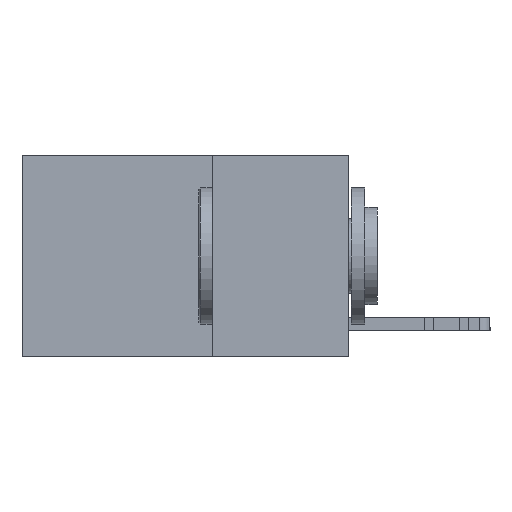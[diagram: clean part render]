
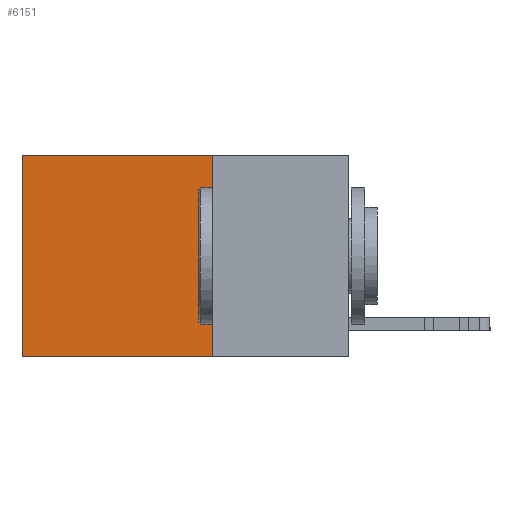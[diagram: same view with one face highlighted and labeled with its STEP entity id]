
A CAD part, left-side view. The second image highlights one B-rep face of the part: STEP entity #6151.
In plain terms, the highlighted planar face has unit normal (-1, 0, 0).
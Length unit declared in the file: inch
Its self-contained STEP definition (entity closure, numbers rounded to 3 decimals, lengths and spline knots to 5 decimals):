
#1271 = VERTEX_POINT ( 'NONE', #16680 ) ;
#1793 = EDGE_CURVE ( 'NONE', #1271, #24748, #17852, .T. ) ;
#2706 = FACE_OUTER_BOUND ( 'NONE', #16881, .T. ) ;
#2847 = VECTOR ( 'NONE', #13712, 39.37008 ) ;
#3685 = CARTESIAN_POINT ( 'NONE',  ( 0.2625, 0.25, -0.37 ) ) ;
#4338 = VECTOR ( 'NONE', #7626, 39.37008 ) ;
#4457 = CARTESIAN_POINT ( 'NONE',  ( 0.2625, 0.25, -0.37 ) ) ;
#5305 = CARTESIAN_POINT ( 'NONE',  ( 0.2625, 0.25, 0. ) ) ;
#6151 = ADVANCED_FACE ( 'NONE', ( #2706 ), #21548, .F. ) ;
#7626 = DIRECTION ( 'NONE',  ( 0., 1., 0. ) ) ;
#8048 = CARTESIAN_POINT ( 'NONE',  ( 0.2625, 0.25, 0. ) ) ;
#8070 = ORIENTED_EDGE ( 'NONE', *, *, #14842, .T. ) ;
#12489 = VERTEX_POINT ( 'NONE', #4457 ) ;
#12623 = DIRECTION ( 'NONE',  ( 0., 0., -1. ) ) ;
#13712 = DIRECTION ( 'NONE',  ( 0., 1., 0. ) ) ;
#14151 = DIRECTION ( 'NONE',  ( 0., 0., -1. ) ) ;
#14467 = AXIS2_PLACEMENT_3D ( 'NONE', #19234, #28657, #14151 ) ;
#14790 = ORIENTED_EDGE ( 'NONE', *, *, #1793, .T. ) ;
#14842 = EDGE_CURVE ( 'NONE', #24601, #1271, #28615, .T. ) ;
#16164 = VECTOR ( 'NONE', #17483, 39.37008 ) ;
#16222 = EDGE_CURVE ( 'NONE', #24601, #12489, #22092, .T. ) ;
#16467 = CARTESIAN_POINT ( 'NONE',  ( 0.2625, 0.25, 0. ) ) ;
#16680 = CARTESIAN_POINT ( 'NONE',  ( 0.2625, 0.6, 0. ) ) ;
#16789 = EDGE_CURVE ( 'NONE', #12489, #24748, #24835, .T. ) ;
#16881 = EDGE_LOOP ( 'NONE', ( #14790, #17646, #28632, #8070 ) ) ;
#17073 = CARTESIAN_POINT ( 'NONE',  ( 0.2625, 0.6, -0.37 ) ) ;
#17483 = DIRECTION ( 'NONE',  ( 0., 0., -1. ) ) ;
#17646 = ORIENTED_EDGE ( 'NONE', *, *, #16789, .F. ) ;
#17852 = LINE ( 'NONE', #19877, #21232 ) ;
#19234 = CARTESIAN_POINT ( 'NONE',  ( 0.2625, 0.25, 0. ) ) ;
#19877 = CARTESIAN_POINT ( 'NONE',  ( 0.2625, 0.6, 0. ) ) ;
#21232 = VECTOR ( 'NONE', #12623, 39.37008 ) ;
#21548 = PLANE ( 'NONE',  #14467 ) ;
#22092 = LINE ( 'NONE', #8048, #16164 ) ;
#24601 = VERTEX_POINT ( 'NONE', #16467 ) ;
#24748 = VERTEX_POINT ( 'NONE', #17073 ) ;
#24835 = LINE ( 'NONE', #3685, #2847 ) ;
#28615 = LINE ( 'NONE', #5305, #4338 ) ;
#28632 = ORIENTED_EDGE ( 'NONE', *, *, #16222, .F. ) ;
#28657 = DIRECTION ( 'NONE',  ( 1., 0., 0. ) ) ;
